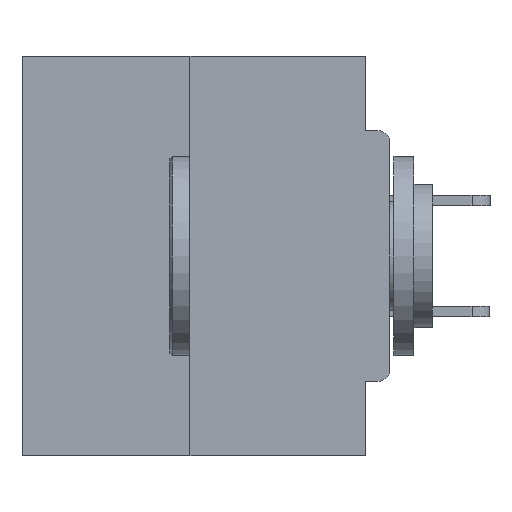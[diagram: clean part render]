
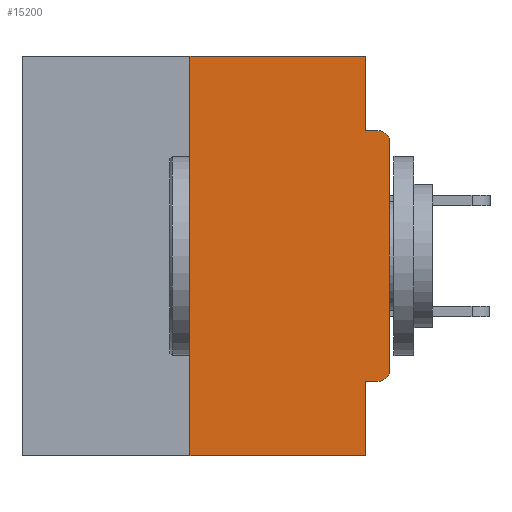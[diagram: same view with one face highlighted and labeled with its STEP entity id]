
A CAD part, left-side view. The second image highlights one B-rep face of the part: STEP entity #15200.
In plain terms, the highlighted planar face has unit normal (-1, 0, 0).
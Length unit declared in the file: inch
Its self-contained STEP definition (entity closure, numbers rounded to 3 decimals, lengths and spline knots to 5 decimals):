
#215 = AXIS2_PLACEMENT_3D ( 'NONE', #2264, #31672, #14161 ) ;
#371 = VECTOR ( 'NONE', #19490, 39.37008 ) ;
#405 = LINE ( 'NONE', #12423, #31929 ) ;
#529 = EDGE_CURVE ( 'NONE', #33284, #18795, #26780, .T. ) ;
#538 = CARTESIAN_POINT ( 'NONE',  ( 0., 0.46, -0.5 ) ) ;
#756 = CARTESIAN_POINT ( 'NONE',  ( 0., 0.015, -0.1085 ) ) ;
#1159 = EDGE_CURVE ( 'NONE', #9329, #27993, #3433, .T. ) ;
#1643 = CARTESIAN_POINT ( 'NONE',  ( 0., 0.031, 0. ) ) ;
#2264 = CARTESIAN_POINT ( 'NONE',  ( 0., 0.015, -0.3915 ) ) ;
#2427 = ORIENTED_EDGE ( 'NONE', *, *, #14625, .T. ) ;
#3000 = CARTESIAN_POINT ( 'NONE',  ( 0., 0.031, 0. ) ) ;
#3283 = DIRECTION ( 'NONE',  ( 0., 0., -1. ) ) ;
#3433 = LINE ( 'NONE', #3000, #8475 ) ;
#4182 = VERTEX_POINT ( 'NONE', #33141 ) ;
#5487 = AXIS2_PLACEMENT_3D ( 'NONE', #11966, #9066, #3283 ) ;
#5571 = VERTEX_POINT ( 'NONE', #12148 ) ;
#5963 = DIRECTION ( 'NONE',  ( 0., 0., -1. ) ) ;
#6064 = CARTESIAN_POINT ( 'NONE',  ( 0., 0.031, -0.0935 ) ) ;
#6772 = EDGE_CURVE ( 'NONE', #30060, #31613, #14113, .T. ) ;
#6925 = DIRECTION ( 'NONE',  ( 0., 0., -1. ) ) ;
#8036 = ORIENTED_EDGE ( 'NONE', *, *, #6772, .T. ) ;
#8085 = EDGE_CURVE ( 'NONE', #5571, #4182, #35052, .T. ) ;
#8475 = VECTOR ( 'NONE', #5963, 39.37008 ) ;
#8884 = CARTESIAN_POINT ( 'NONE',  ( 0., 0.25, -0.5 ) ) ;
#8980 = CARTESIAN_POINT ( 'NONE',  ( 0., 0., -0.0935 ) ) ;
#9066 = DIRECTION ( 'NONE',  ( 1., 0., 0. ) ) ;
#9329 = VERTEX_POINT ( 'NONE', #1643 ) ;
#9527 = LINE ( 'NONE', #22278, #371 ) ;
#9852 = ORIENTED_EDGE ( 'NONE', *, *, #25795, .F. ) ;
#10588 = ORIENTED_EDGE ( 'NONE', *, *, #14240, .F. ) ;
#11966 = CARTESIAN_POINT ( 'NONE',  ( 0., 0.46, 0. ) ) ;
#12148 = CARTESIAN_POINT ( 'NONE',  ( 0., 0., -0.1085 ) ) ;
#12423 = CARTESIAN_POINT ( 'NONE',  ( 0., 0.46, 0. ) ) ;
#12603 = VECTOR ( 'NONE', #19402, 39.37008 ) ;
#13646 = LINE ( 'NONE', #8980, #14588 ) ;
#13787 = VERTEX_POINT ( 'NONE', #26592 ) ;
#14113 = LINE ( 'NONE', #538, #20978 ) ;
#14161 = DIRECTION ( 'NONE',  ( 0., 0., -1. ) ) ;
#14240 = EDGE_CURVE ( 'NONE', #30060, #26049, #22421, .T. ) ;
#14588 = VECTOR ( 'NONE', #23373, 39.37008 ) ;
#14625 = EDGE_CURVE ( 'NONE', #18795, #5571, #34248, .T. ) ;
#14628 = CARTESIAN_POINT ( 'NONE',  ( 0., 0.25, 0. ) ) ;
#14695 = EDGE_LOOP ( 'NONE', ( #16848, #10588, #8036, #33343, #9852, #31494, #2427, #22167, #33524, #19000 ) ) ;
#15200 = ADVANCED_FACE ( 'NONE', ( #29292 ), #23331, .F. ) ;
#16848 = ORIENTED_EDGE ( 'NONE', *, *, #37219, .F. ) ;
#16975 = EDGE_CURVE ( 'NONE', #13787, #31613, #20861, .T. ) ;
#17933 = CARTESIAN_POINT ( 'NONE',  ( 0., 0., -0.3915 ) ) ;
#18784 = VECTOR ( 'NONE', #23484, 39.37008 ) ;
#18795 = VERTEX_POINT ( 'NONE', #17933 ) ;
#19000 = ORIENTED_EDGE ( 'NONE', *, *, #1159, .F. ) ;
#19402 = DIRECTION ( 'NONE',  ( 0., 0., -1. ) ) ;
#19490 = DIRECTION ( 'NONE',  ( 0., 1., 0. ) ) ;
#20576 = VECTOR ( 'NONE', #22834, 39.37008 ) ;
#20861 = LINE ( 'NONE', #36818, #12603 ) ;
#20978 = VECTOR ( 'NONE', #26969, 39.37008 ) ;
#22167 = ORIENTED_EDGE ( 'NONE', *, *, #8085, .T. ) ;
#22278 = CARTESIAN_POINT ( 'NONE',  ( 0., 0., -0.4065 ) ) ;
#22421 = LINE ( 'NONE', #26170, #18784 ) ;
#22834 = DIRECTION ( 'NONE',  ( 0., 0., 1. ) ) ;
#23331 = PLANE ( 'NONE',  #5487 ) ;
#23373 = DIRECTION ( 'NONE',  ( 0., -1., 0. ) ) ;
#23484 = DIRECTION ( 'NONE',  ( 0., 0., 1. ) ) ;
#25095 = EDGE_CURVE ( 'NONE', #27993, #4182, #13646, .T. ) ;
#25140 = CARTESIAN_POINT ( 'NONE',  ( 0., 0., 0. ) ) ;
#25795 = EDGE_CURVE ( 'NONE', #33284, #13787, #9527, .T. ) ;
#25899 = CARTESIAN_POINT ( 'NONE',  ( 0., 0.015, -0.4065 ) ) ;
#26049 = VERTEX_POINT ( 'NONE', #14628 ) ;
#26170 = CARTESIAN_POINT ( 'NONE',  ( 0., 0.25, 0. ) ) ;
#26592 = CARTESIAN_POINT ( 'NONE',  ( 0., 0.031, -0.4065 ) ) ;
#26780 = CIRCLE ( 'NONE', #215, 0.015 ) ;
#26969 = DIRECTION ( 'NONE',  ( 0., -1., 0. ) ) ;
#27993 = VERTEX_POINT ( 'NONE', #6064 ) ;
#29292 = FACE_OUTER_BOUND ( 'NONE', #14695, .T. ) ;
#29658 = CARTESIAN_POINT ( 'NONE',  ( 0., 0.031, -0.5 ) ) ;
#30060 = VERTEX_POINT ( 'NONE', #8884 ) ;
#31494 = ORIENTED_EDGE ( 'NONE', *, *, #529, .T. ) ;
#31613 = VERTEX_POINT ( 'NONE', #29658 ) ;
#31672 = DIRECTION ( 'NONE',  ( -1., 0., 0. ) ) ;
#31929 = VECTOR ( 'NONE', #32876, 39.37008 ) ;
#32831 = DIRECTION ( 'NONE',  ( -1., 0., 0. ) ) ;
#32876 = DIRECTION ( 'NONE',  ( 0., -1., 0. ) ) ;
#33141 = CARTESIAN_POINT ( 'NONE',  ( 0., 0.015, -0.0935 ) ) ;
#33284 = VERTEX_POINT ( 'NONE', #25899 ) ;
#33343 = ORIENTED_EDGE ( 'NONE', *, *, #16975, .F. ) ;
#33524 = ORIENTED_EDGE ( 'NONE', *, *, #25095, .F. ) ;
#34248 = LINE ( 'NONE', #25140, #20576 ) ;
#34856 = AXIS2_PLACEMENT_3D ( 'NONE', #756, #32831, #6925 ) ;
#35052 = CIRCLE ( 'NONE', #34856, 0.015 ) ;
#36818 = CARTESIAN_POINT ( 'NONE',  ( 0., 0.031, -0.5 ) ) ;
#37219 = EDGE_CURVE ( 'NONE', #26049, #9329, #405, .T. ) ;
